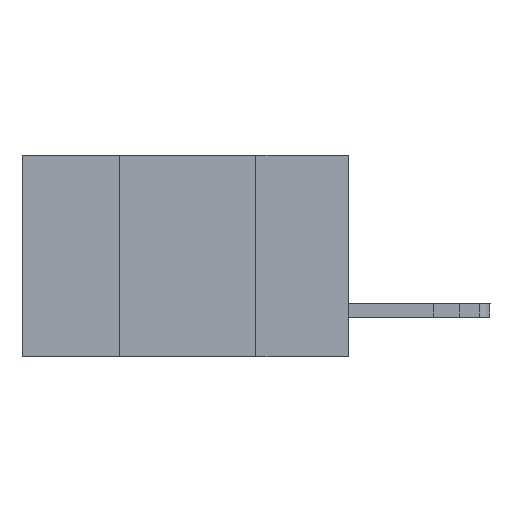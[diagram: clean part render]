
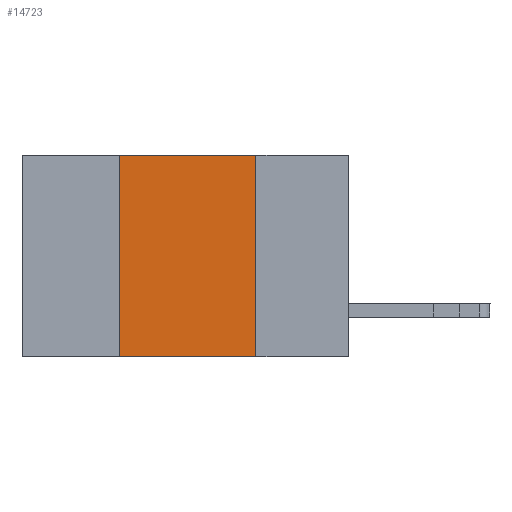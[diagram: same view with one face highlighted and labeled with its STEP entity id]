
A CAD part, left-side view. The second image highlights one B-rep face of the part: STEP entity #14723.
In plain terms, the highlighted planar face has unit normal (-1, 0, 0).
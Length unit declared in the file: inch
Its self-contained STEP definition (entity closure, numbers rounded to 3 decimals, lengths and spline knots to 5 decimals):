
#145 = CARTESIAN_POINT ( 'NONE',  ( 0., 0.17, -0.37 ) ) ;
#385 = FACE_OUTER_BOUND ( 'NONE', #734, .T. ) ;
#734 = EDGE_LOOP ( 'NONE', ( #3721, #8322, #2922, #14303 ) ) ;
#1066 = LINE ( 'NONE', #3045, #1095 ) ;
#1095 = VECTOR ( 'NONE', #9166, 39.37008 ) ;
#1381 = VERTEX_POINT ( 'NONE', #6143 ) ;
#1718 = LINE ( 'NONE', #6466, #9491 ) ;
#1987 = CARTESIAN_POINT ( 'NONE',  ( 0., 0.42, -0.37 ) ) ;
#2631 = DIRECTION ( 'NONE',  ( 0., -1., 0. ) ) ;
#2922 = ORIENTED_EDGE ( 'NONE', *, *, #7878, .F. ) ;
#3045 = CARTESIAN_POINT ( 'NONE',  ( 0., 0.42, -0.37 ) ) ;
#3321 = VECTOR ( 'NONE', #2631, 39.37008 ) ;
#3721 = ORIENTED_EDGE ( 'NONE', *, *, #6039, .F. ) ;
#3972 = CARTESIAN_POINT ( 'NONE',  ( 0., 0.17, -0.37 ) ) ;
#4536 = AXIS2_PLACEMENT_3D ( 'NONE', #11597, #12902, #13962 ) ;
#6039 = EDGE_CURVE ( 'NONE', #12174, #10663, #9598, .T. ) ;
#6143 = CARTESIAN_POINT ( 'NONE',  ( 0., 0.42, 0. ) ) ;
#6466 = CARTESIAN_POINT ( 'NONE',  ( 0., 0.6, 0. ) ) ;
#7878 = EDGE_CURVE ( 'NONE', #14361, #1381, #1066, .T. ) ;
#8322 = ORIENTED_EDGE ( 'NONE', *, *, #10657, .F. ) ;
#9166 = DIRECTION ( 'NONE',  ( 0., 0., 1. ) ) ;
#9491 = VECTOR ( 'NONE', #11203, 39.37008 ) ;
#9598 = LINE ( 'NONE', #145, #14271 ) ;
#10439 = DIRECTION ( 'NONE',  ( 0., 0., -1. ) ) ;
#10657 = EDGE_CURVE ( 'NONE', #1381, #12174, #1718, .T. ) ;
#10663 = VERTEX_POINT ( 'NONE', #3972 ) ;
#11203 = DIRECTION ( 'NONE',  ( 0., -1., 0. ) ) ;
#11597 = CARTESIAN_POINT ( 'NONE',  ( 0., 0.6, 0. ) ) ;
#11904 = PLANE ( 'NONE',  #4536 ) ;
#12174 = VERTEX_POINT ( 'NONE', #14592 ) ;
#12642 = EDGE_CURVE ( 'NONE', #14361, #10663, #12977, .T. ) ;
#12736 = CARTESIAN_POINT ( 'NONE',  ( 0., 0.6, -0.37 ) ) ;
#12902 = DIRECTION ( 'NONE',  ( 1., 0., 0. ) ) ;
#12977 = LINE ( 'NONE', #12736, #3321 ) ;
#13962 = DIRECTION ( 'NONE',  ( 0., 0., -1. ) ) ;
#14271 = VECTOR ( 'NONE', #10439, 39.37008 ) ;
#14303 = ORIENTED_EDGE ( 'NONE', *, *, #12642, .T. ) ;
#14361 = VERTEX_POINT ( 'NONE', #1987 ) ;
#14592 = CARTESIAN_POINT ( 'NONE',  ( 0., 0.17, 0. ) ) ;
#14723 = ADVANCED_FACE ( 'NONE', ( #385 ), #11904, .F. ) ;
